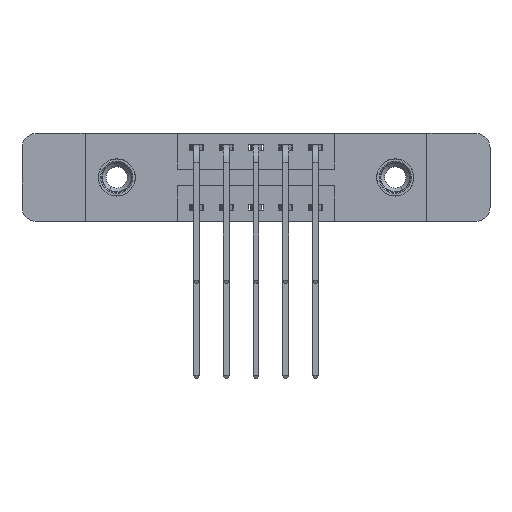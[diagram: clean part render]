
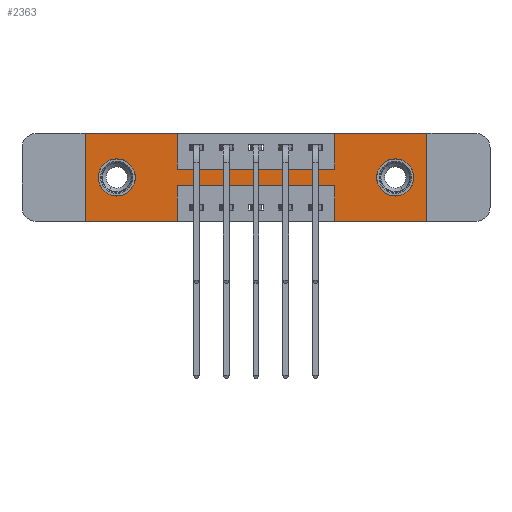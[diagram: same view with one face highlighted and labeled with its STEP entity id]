
A CAD part, front view. The second image highlights one B-rep face of the part: STEP entity #2363.
In plain terms, the highlighted planar face has unit normal (0, -1, 0).
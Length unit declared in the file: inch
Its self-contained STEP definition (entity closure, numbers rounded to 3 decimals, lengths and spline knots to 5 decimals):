
#118 = LINE ( 'NONE', #4967, #14563 ) ;
#194 = DIRECTION ( 'NONE',  ( -1., 0., 0. ) ) ;
#274 = LINE ( 'NONE', #7349, #8370 ) ;
#295 = VERTEX_POINT ( 'NONE', #2513 ) ;
#376 = EDGE_CURVE ( 'NONE', #7290, #1148, #274, .T. ) ;
#778 = DIRECTION ( 'NONE',  ( 0., 1., 0. ) ) ;
#803 = ORIENTED_EDGE ( 'NONE', *, *, #10029, .T. ) ;
#813 = VECTOR ( 'NONE', #9064, 39.37008 ) ;
#930 = CARTESIAN_POINT ( 'NONE',  ( 1.3025, 0., -0.185 ) ) ;
#1018 = VERTEX_POINT ( 'NONE', #14667 ) ;
#1034 = EDGE_CURVE ( 'NONE', #3064, #15195, #7099, .T. ) ;
#1148 = VERTEX_POINT ( 'NONE', #11248 ) ;
#1317 = AXIS2_PLACEMENT_3D ( 'NONE', #2603, #13743, #7438 ) ;
#1346 = ORIENTED_EDGE ( 'NONE', *, *, #6364, .F. ) ;
#1482 = ORIENTED_EDGE ( 'NONE', *, *, #8007, .F. ) ;
#1599 = DIRECTION ( 'NONE',  ( 0., 0., -1. ) ) ;
#2363 = ADVANCED_FACE ( 'NONE', ( #14573, #3739, #8403 ), #2538, .T. ) ;
#2458 = ORIENTED_EDGE ( 'NONE', *, *, #12832, .F. ) ;
#2513 = CARTESIAN_POINT ( 'NONE',  ( 0.3875, 0., -0.15 ) ) ;
#2538 = PLANE ( 'NONE',  #7385 ) ;
#2603 = CARTESIAN_POINT ( 'NONE',  ( 0.1325, 0., -0.185 ) ) ;
#2830 = EDGE_CURVE ( 'NONE', #6395, #5449, #3563, .T. ) ;
#2975 = CARTESIAN_POINT ( 'NONE',  ( 1.0475, 0., 0. ) ) ;
#3064 = VERTEX_POINT ( 'NONE', #11438 ) ;
#3233 = ORIENTED_EDGE ( 'NONE', *, *, #2830, .F. ) ;
#3513 = LINE ( 'NONE', #14414, #10543 ) ;
#3563 = LINE ( 'NONE', #8384, #15459 ) ;
#3739 = FACE_BOUND ( 'NONE', #14480, .T. ) ;
#3753 = CARTESIAN_POINT ( 'NONE',  ( 0.3875, 0., 0. ) ) ;
#3811 = CARTESIAN_POINT ( 'NONE',  ( 0., 0., -0.37 ) ) ;
#3825 = ORIENTED_EDGE ( 'NONE', *, *, #1034, .T. ) ;
#3912 = DIRECTION ( 'NONE',  ( 0., 1., 0. ) ) ;
#4164 = VERTEX_POINT ( 'NONE', #14918 ) ;
#4204 = DIRECTION ( 'NONE',  ( 1., 0., 0. ) ) ;
#4226 = VECTOR ( 'NONE', #4204, 39.37008 ) ;
#4558 = EDGE_LOOP ( 'NONE', ( #3825, #803 ) ) ;
#4589 = LINE ( 'NONE', #11927, #6156 ) ;
#4693 = VERTEX_POINT ( 'NONE', #6915 ) ;
#4742 = CARTESIAN_POINT ( 'NONE',  ( 0., 0., -0.37 ) ) ;
#4828 = CARTESIAN_POINT ( 'NONE',  ( 1.0475, 0., 0. ) ) ;
#4967 = CARTESIAN_POINT ( 'NONE',  ( 0.3875, 0., -0.22 ) ) ;
#5078 = ORIENTED_EDGE ( 'NONE', *, *, #11099, .T. ) ;
#5175 = LINE ( 'NONE', #9997, #5910 ) ;
#5204 = VERTEX_POINT ( 'NONE', #14080 ) ;
#5449 = VERTEX_POINT ( 'NONE', #12551 ) ;
#5571 = EDGE_CURVE ( 'NONE', #1018, #295, #13393, .T. ) ;
#5782 = DIRECTION ( 'NONE',  ( 0., 1., 0. ) ) ;
#5910 = VECTOR ( 'NONE', #14824, 39.37008 ) ;
#5950 = ORIENTED_EDGE ( 'NONE', *, *, #13528, .F. ) ;
#6056 = EDGE_LOOP ( 'NONE', ( #9663, #5950, #7798, #14795, #1346, #3233, #1482, #2458, #11758, #7390, #10782, #10628 ) ) ;
#6156 = VECTOR ( 'NONE', #15645, 39.37008 ) ;
#6364 = EDGE_CURVE ( 'NONE', #5449, #13083, #4589, .T. ) ;
#6392 = VERTEX_POINT ( 'NONE', #10752 ) ;
#6395 = VERTEX_POINT ( 'NONE', #4828 ) ;
#6576 = LINE ( 'NONE', #11379, #4226 ) ;
#6610 = CARTESIAN_POINT ( 'NONE',  ( 0., 0., 0. ) ) ;
#6856 = CARTESIAN_POINT ( 'NONE',  ( 1.3025, 0., -0.263 ) ) ;
#6915 = CARTESIAN_POINT ( 'NONE',  ( 0., 0., -0.37 ) ) ;
#7099 = CIRCLE ( 'NONE', #12138, 0.078 ) ;
#7290 = VERTEX_POINT ( 'NONE', #10756 ) ;
#7349 = CARTESIAN_POINT ( 'NONE',  ( 1.0475, 0., -0.37 ) ) ;
#7385 = AXIS2_PLACEMENT_3D ( 'NONE', #3811, #13233, #12193 ) ;
#7390 = ORIENTED_EDGE ( 'NONE', *, *, #15163, .F. ) ;
#7410 = EDGE_CURVE ( 'NONE', #4164, #11454, #13699, .T. ) ;
#7438 = DIRECTION ( 'NONE',  ( 0., 0., 1. ) ) ;
#7699 = EDGE_CURVE ( 'NONE', #12279, #4693, #9474, .T. ) ;
#7792 = LINE ( 'NONE', #6610, #11949 ) ;
#7798 = ORIENTED_EDGE ( 'NONE', *, *, #376, .F. ) ;
#7865 = LINE ( 'NONE', #2975, #813 ) ;
#7954 = EDGE_CURVE ( 'NONE', #4693, #15626, #7792, .T. ) ;
#8007 = EDGE_CURVE ( 'NONE', #5204, #6395, #7865, .T. ) ;
#8038 = DIRECTION ( 'NONE',  ( 1., 0., 0. ) ) ;
#8370 = VECTOR ( 'NONE', #14856, 39.37008 ) ;
#8375 = EDGE_CURVE ( 'NONE', #13083, #7290, #5175, .T. ) ;
#8384 = CARTESIAN_POINT ( 'NONE',  ( 0., 0., 0. ) ) ;
#8403 = FACE_OUTER_BOUND ( 'NONE', #6056, .T. ) ;
#9033 = CARTESIAN_POINT ( 'NONE',  ( 1.3025, 0., -0.185 ) ) ;
#9064 = DIRECTION ( 'NONE',  ( 0., 0., 1. ) ) ;
#9474 = LINE ( 'NONE', #4742, #12202 ) ;
#9663 = ORIENTED_EDGE ( 'NONE', *, *, #14423, .F. ) ;
#9730 = CARTESIAN_POINT ( 'NONE',  ( 1.435, 0., -0.37 ) ) ;
#9997 = CARTESIAN_POINT ( 'NONE',  ( 0., 0., -0.37 ) ) ;
#10029 = EDGE_CURVE ( 'NONE', #15195, #3064, #14531, .T. ) ;
#10543 = VECTOR ( 'NONE', #10936, 39.37008 ) ;
#10628 = ORIENTED_EDGE ( 'NONE', *, *, #7699, .F. ) ;
#10739 = DIRECTION ( 'NONE',  ( -1., 0., 0. ) ) ;
#10752 = CARTESIAN_POINT ( 'NONE',  ( 0.3875, 0., -0.22 ) ) ;
#10756 = CARTESIAN_POINT ( 'NONE',  ( 1.0475, 0., -0.37 ) ) ;
#10782 = ORIENTED_EDGE ( 'NONE', *, *, #7954, .F. ) ;
#10936 = DIRECTION ( 'NONE',  ( 0., 0., -1. ) ) ;
#10944 = DIRECTION ( 'NONE',  ( 0., 0., -1. ) ) ;
#11003 = CIRCLE ( 'NONE', #15302, 0.078 ) ;
#11051 = VECTOR ( 'NONE', #8038, 39.37008 ) ;
#11099 = EDGE_CURVE ( 'NONE', #11454, #4164, #11003, .T. ) ;
#11248 = CARTESIAN_POINT ( 'NONE',  ( 1.0475, 0., -0.22 ) ) ;
#11379 = CARTESIAN_POINT ( 'NONE',  ( 0.3875, 0., -0.15 ) ) ;
#11438 = CARTESIAN_POINT ( 'NONE',  ( 1.3025, 0., -0.107 ) ) ;
#11454 = VERTEX_POINT ( 'NONE', #14948 ) ;
#11758 = ORIENTED_EDGE ( 'NONE', *, *, #5571, .F. ) ;
#11927 = CARTESIAN_POINT ( 'NONE',  ( 1.435, 0., 0. ) ) ;
#11949 = VECTOR ( 'NONE', #14994, 39.37008 ) ;
#12077 = CARTESIAN_POINT ( 'NONE',  ( 0.3875, 0., -0.37 ) ) ;
#12138 = AXIS2_PLACEMENT_3D ( 'NONE', #930, #5782, #1599 ) ;
#12193 = DIRECTION ( 'NONE',  ( 0., 0., -1. ) ) ;
#12202 = VECTOR ( 'NONE', #10739, 39.37008 ) ;
#12244 = AXIS2_PLACEMENT_3D ( 'NONE', #9033, #778, #15270 ) ;
#12279 = VERTEX_POINT ( 'NONE', #12077 ) ;
#12551 = CARTESIAN_POINT ( 'NONE',  ( 1.435, 0., 0. ) ) ;
#12832 = EDGE_CURVE ( 'NONE', #295, #5204, #6576, .T. ) ;
#13083 = VERTEX_POINT ( 'NONE', #9730 ) ;
#13211 = DIRECTION ( 'NONE',  ( 1., 0., 0. ) ) ;
#13233 = DIRECTION ( 'NONE',  ( 0., -1., 0. ) ) ;
#13393 = LINE ( 'NONE', #3753, #15469 ) ;
#13528 = EDGE_CURVE ( 'NONE', #1148, #6392, #118, .T. ) ;
#13699 = CIRCLE ( 'NONE', #1317, 0.078 ) ;
#13743 = DIRECTION ( 'NONE',  ( 0., 1., 0. ) ) ;
#13778 = DIRECTION ( 'NONE',  ( 0., 0., 1. ) ) ;
#13853 = CARTESIAN_POINT ( 'NONE',  ( 0.1325, 0., -0.185 ) ) ;
#14080 = CARTESIAN_POINT ( 'NONE',  ( 1.0475, 0., -0.15 ) ) ;
#14104 = CARTESIAN_POINT ( 'NONE',  ( 0., 0., 0. ) ) ;
#14283 = LINE ( 'NONE', #14433, #11051 ) ;
#14414 = CARTESIAN_POINT ( 'NONE',  ( 0.3875, 0., -0.37 ) ) ;
#14423 = EDGE_CURVE ( 'NONE', #6392, #12279, #3513, .T. ) ;
#14433 = CARTESIAN_POINT ( 'NONE',  ( 0., 0., 0. ) ) ;
#14480 = EDGE_LOOP ( 'NONE', ( #15138, #5078 ) ) ;
#14531 = CIRCLE ( 'NONE', #12244, 0.078 ) ;
#14563 = VECTOR ( 'NONE', #194, 39.37008 ) ;
#14573 = FACE_BOUND ( 'NONE', #4558, .T. ) ;
#14667 = CARTESIAN_POINT ( 'NONE',  ( 0.3875, 0., 0. ) ) ;
#14795 = ORIENTED_EDGE ( 'NONE', *, *, #8375, .F. ) ;
#14824 = DIRECTION ( 'NONE',  ( -1., 0., 0. ) ) ;
#14856 = DIRECTION ( 'NONE',  ( 0., 0., 1. ) ) ;
#14918 = CARTESIAN_POINT ( 'NONE',  ( 0.1325, 0., -0.107 ) ) ;
#14948 = CARTESIAN_POINT ( 'NONE',  ( 0.1325, 0., -0.263 ) ) ;
#14994 = DIRECTION ( 'NONE',  ( 0., 0., 1. ) ) ;
#15138 = ORIENTED_EDGE ( 'NONE', *, *, #7410, .T. ) ;
#15163 = EDGE_CURVE ( 'NONE', #15626, #1018, #14283, .T. ) ;
#15195 = VERTEX_POINT ( 'NONE', #6856 ) ;
#15270 = DIRECTION ( 'NONE',  ( 0., 0., -1. ) ) ;
#15302 = AXIS2_PLACEMENT_3D ( 'NONE', #13853, #3912, #13778 ) ;
#15459 = VECTOR ( 'NONE', #13211, 39.37008 ) ;
#15469 = VECTOR ( 'NONE', #10944, 39.37008 ) ;
#15626 = VERTEX_POINT ( 'NONE', #14104 ) ;
#15645 = DIRECTION ( 'NONE',  ( 0., 0., -1. ) ) ;
